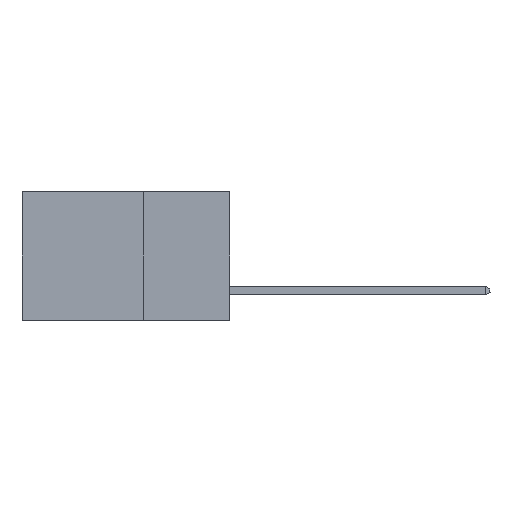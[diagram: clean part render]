
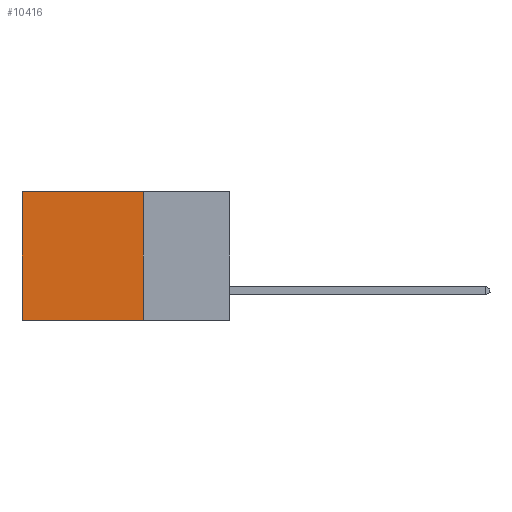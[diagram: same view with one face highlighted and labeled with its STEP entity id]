
A CAD part, left-side view. The second image highlights one B-rep face of the part: STEP entity #10416.
In plain terms, the highlighted planar face has unit normal (-1, 0, 0).
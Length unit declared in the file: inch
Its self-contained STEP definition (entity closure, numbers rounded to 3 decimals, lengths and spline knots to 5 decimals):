
#477 = CARTESIAN_POINT ( 'NONE',  ( 0.298, 0.6, -0.37 ) ) ;
#757 = VERTEX_POINT ( 'NONE', #2537 ) ;
#984 = CARTESIAN_POINT ( 'NONE',  ( 0.298, 0.25, 0. ) ) ;
#1167 = DIRECTION ( 'NONE',  ( 1., 0., 0. ) ) ;
#1761 = VECTOR ( 'NONE', #8019, 39.37008 ) ;
#1995 = ORIENTED_EDGE ( 'NONE', *, *, #8189, .T. ) ;
#2358 = CARTESIAN_POINT ( 'NONE',  ( 0.298, 0.25, -0.37 ) ) ;
#2537 = CARTESIAN_POINT ( 'NONE',  ( 0.298, 0.25, 0. ) ) ;
#2719 = EDGE_CURVE ( 'NONE', #757, #8558, #7734, .T. ) ;
#2752 = AXIS2_PLACEMENT_3D ( 'NONE', #7164, #1167, #10368 ) ;
#2937 = VERTEX_POINT ( 'NONE', #6777 ) ;
#4015 = DIRECTION ( 'NONE',  ( 0., 1., 0. ) ) ;
#4733 = VERTEX_POINT ( 'NONE', #477 ) ;
#5025 = CARTESIAN_POINT ( 'NONE',  ( 0.298, 0.25, 0. ) ) ;
#5162 = FACE_OUTER_BOUND ( 'NONE', #8953, .T. ) ;
#5913 = CARTESIAN_POINT ( 'NONE',  ( 0.298, 0.25, -0.37 ) ) ;
#6213 = VECTOR ( 'NONE', #9990, 39.37008 ) ;
#6600 = CARTESIAN_POINT ( 'NONE',  ( 0.298, 0.6, 0. ) ) ;
#6777 = CARTESIAN_POINT ( 'NONE',  ( 0.298, 0.6, 0. ) ) ;
#6922 = ORIENTED_EDGE ( 'NONE', *, *, #11405, .F. ) ;
#7140 = LINE ( 'NONE', #5913, #6213 ) ;
#7164 = CARTESIAN_POINT ( 'NONE',  ( 0.298, 0.25, 0. ) ) ;
#7237 = LINE ( 'NONE', #6600, #8779 ) ;
#7300 = EDGE_CURVE ( 'NONE', #2937, #4733, #7237, .T. ) ;
#7734 = LINE ( 'NONE', #5025, #1761 ) ;
#8019 = DIRECTION ( 'NONE',  ( 0., 0., -1. ) ) ;
#8168 = PLANE ( 'NONE',  #2752 ) ;
#8189 = EDGE_CURVE ( 'NONE', #757, #2937, #8456, .T. ) ;
#8291 = ORIENTED_EDGE ( 'NONE', *, *, #7300, .T. ) ;
#8456 = LINE ( 'NONE', #984, #11997 ) ;
#8558 = VERTEX_POINT ( 'NONE', #2358 ) ;
#8596 = DIRECTION ( 'NONE',  ( 0., 0., -1. ) ) ;
#8779 = VECTOR ( 'NONE', #8596, 39.37008 ) ;
#8789 = ORIENTED_EDGE ( 'NONE', *, *, #2719, .F. ) ;
#8953 = EDGE_LOOP ( 'NONE', ( #8291, #6922, #8789, #1995 ) ) ;
#9990 = DIRECTION ( 'NONE',  ( 0., 1., 0. ) ) ;
#10368 = DIRECTION ( 'NONE',  ( 0., 0., -1. ) ) ;
#10416 = ADVANCED_FACE ( 'NONE', ( #5162 ), #8168, .F. ) ;
#11405 = EDGE_CURVE ( 'NONE', #8558, #4733, #7140, .T. ) ;
#11997 = VECTOR ( 'NONE', #4015, 39.37008 ) ;
